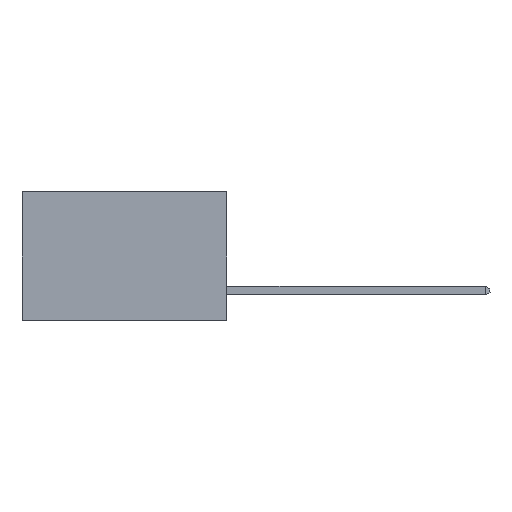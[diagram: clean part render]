
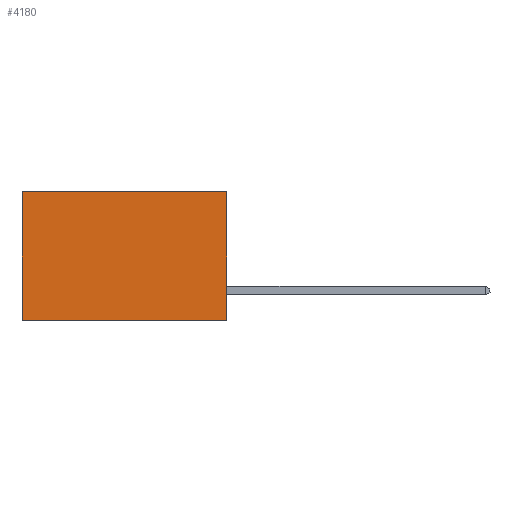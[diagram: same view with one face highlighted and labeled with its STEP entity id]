
A CAD part, left-side view. The second image highlights one B-rep face of the part: STEP entity #4180.
In plain terms, the highlighted planar face has unit normal (-1, 0, 0).
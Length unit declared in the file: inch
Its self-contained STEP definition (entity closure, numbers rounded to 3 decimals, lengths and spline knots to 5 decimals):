
#11 = CARTESIAN_POINT ( 'NONE',  ( 0.277, 0., -0.37 ) ) ;
#576 = VECTOR ( 'NONE', #7535, 39.37008 ) ;
#1327 = VERTEX_POINT ( 'NONE', #7004 ) ;
#1608 = ORIENTED_EDGE ( 'NONE', *, *, #4062, .F. ) ;
#2152 = CARTESIAN_POINT ( 'NONE',  ( 0.277, 0.59, -0.37 ) ) ;
#2781 = DIRECTION ( 'NONE',  ( 0., 0., -1. ) ) ;
#2784 = CARTESIAN_POINT ( 'NONE',  ( 0.277, 0.59, -0.37 ) ) ;
#2801 = VERTEX_POINT ( 'NONE', #7567 ) ;
#2979 = LINE ( 'NONE', #11, #576 ) ;
#3568 = ORIENTED_EDGE ( 'NONE', *, *, #3915, .T. ) ;
#3915 = EDGE_CURVE ( 'NONE', #5234, #9267, #5443, .T. ) ;
#3970 = VECTOR ( 'NONE', #5132, 39.37008 ) ;
#4062 = EDGE_CURVE ( 'NONE', #2801, #1327, #2979, .T. ) ;
#4180 = ADVANCED_FACE ( 'NONE', ( #7788 ), #5090, .F. ) ;
#4347 = CARTESIAN_POINT ( 'NONE',  ( 0.277, 0., -0.37 ) ) ;
#4514 = EDGE_CURVE ( 'NONE', #2801, #5234, #7571, .T. ) ;
#4551 = CARTESIAN_POINT ( 'NONE',  ( 0.277, 0., -0.37 ) ) ;
#5048 = DIRECTION ( 'NONE',  ( 1., 0., 0. ) ) ;
#5090 = PLANE ( 'NONE',  #7303 ) ;
#5132 = DIRECTION ( 'NONE',  ( 0., 1., 0. ) ) ;
#5234 = VERTEX_POINT ( 'NONE', #9154 ) ;
#5443 = LINE ( 'NONE', #2784, #9200 ) ;
#5599 = EDGE_CURVE ( 'NONE', #1327, #9267, #6202, .T. ) ;
#5650 = VECTOR ( 'NONE', #9874, 39.37008 ) ;
#5713 = DIRECTION ( 'NONE',  ( 0., 0., -1. ) ) ;
#5855 = ORIENTED_EDGE ( 'NONE', *, *, #4514, .T. ) ;
#5993 = EDGE_LOOP ( 'NONE', ( #3568, #9369, #1608, #5855 ) ) ;
#6202 = LINE ( 'NONE', #4347, #3970 ) ;
#7004 = CARTESIAN_POINT ( 'NONE',  ( 0.277, 0., -0.37 ) ) ;
#7303 = AXIS2_PLACEMENT_3D ( 'NONE', #4551, #5048, #5713 ) ;
#7535 = DIRECTION ( 'NONE',  ( 0., 0., -1. ) ) ;
#7567 = CARTESIAN_POINT ( 'NONE',  ( 0.277, 0., 0. ) ) ;
#7571 = LINE ( 'NONE', #8544, #5650 ) ;
#7788 = FACE_OUTER_BOUND ( 'NONE', #5993, .T. ) ;
#8544 = CARTESIAN_POINT ( 'NONE',  ( 0.277, 0., 0. ) ) ;
#9154 = CARTESIAN_POINT ( 'NONE',  ( 0.277, 0.59, 0. ) ) ;
#9200 = VECTOR ( 'NONE', #2781, 39.37008 ) ;
#9267 = VERTEX_POINT ( 'NONE', #2152 ) ;
#9369 = ORIENTED_EDGE ( 'NONE', *, *, #5599, .F. ) ;
#9874 = DIRECTION ( 'NONE',  ( 0., 1., 0. ) ) ;
